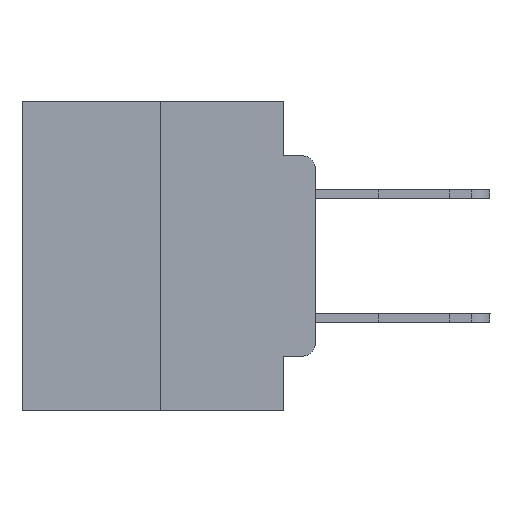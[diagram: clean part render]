
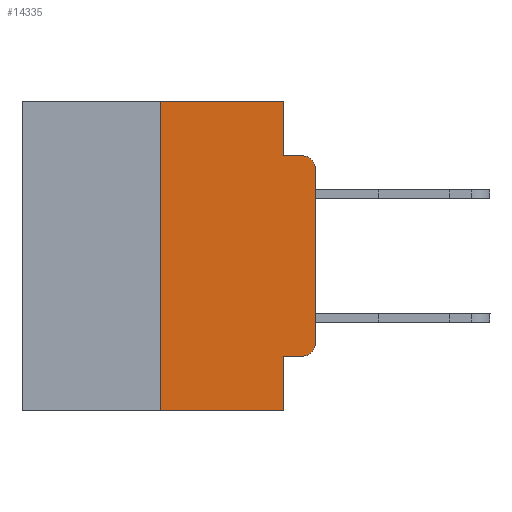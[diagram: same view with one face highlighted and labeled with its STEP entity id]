
A CAD part, left-side view. The second image highlights one B-rep face of the part: STEP entity #14335.
In plain terms, the highlighted planar face has unit normal (-1, 0, 0).
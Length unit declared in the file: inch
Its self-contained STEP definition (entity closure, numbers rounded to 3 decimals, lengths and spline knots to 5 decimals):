
#301 = CARTESIAN_POINT ( 'NONE',  ( 0., 0.051, -0.0885 ) ) ;
#1050 = CARTESIAN_POINT ( 'NONE',  ( 0., 0.02, -0.4115 ) ) ;
#1222 = DIRECTION ( 'NONE',  ( 0., -1., 0. ) ) ;
#1786 = VERTEX_POINT ( 'NONE', #24071 ) ;
#1843 = CARTESIAN_POINT ( 'NONE',  ( 0., 0.473, 0. ) ) ;
#1977 = ORIENTED_EDGE ( 'NONE', *, *, #16049, .F. ) ;
#2689 = LINE ( 'NONE', #21723, #15384 ) ;
#3329 = CARTESIAN_POINT ( 'NONE',  ( 0., 0.25, -0.5 ) ) ;
#3338 = DIRECTION ( 'NONE',  ( -1., 0., 0. ) ) ;
#4397 = VERTEX_POINT ( 'NONE', #22391 ) ;
#4562 = VERTEX_POINT ( 'NONE', #12631 ) ;
#4757 = VERTEX_POINT ( 'NONE', #17362 ) ;
#5115 = DIRECTION ( 'NONE',  ( 0., 0., -1. ) ) ;
#5194 = CARTESIAN_POINT ( 'NONE',  ( 0., 0.473, 0. ) ) ;
#5506 = EDGE_CURVE ( 'NONE', #17036, #4397, #13467, .T. ) ;
#5557 = CARTESIAN_POINT ( 'NONE',  ( 0., 0.25, 0. ) ) ;
#5837 = CARTESIAN_POINT ( 'NONE',  ( 0., 0.051, -0.4115 ) ) ;
#5929 = CARTESIAN_POINT ( 'NONE',  ( 0., 0.02, -0.1085 ) ) ;
#6880 = VECTOR ( 'NONE', #12243, 39.37008 ) ;
#7195 = CARTESIAN_POINT ( 'NONE',  ( 0., 0.25, 0. ) ) ;
#8250 = ORIENTED_EDGE ( 'NONE', *, *, #23955, .T. ) ;
#8496 = CARTESIAN_POINT ( 'NONE',  ( 0., 0.051, 0. ) ) ;
#9149 = AXIS2_PLACEMENT_3D ( 'NONE', #1843, #12012, #22225 ) ;
#9282 = VERTEX_POINT ( 'NONE', #17392 ) ;
#9330 = CARTESIAN_POINT ( 'NONE',  ( 0., 0.02, -0.0885 ) ) ;
#10525 = VECTOR ( 'NONE', #16918, 39.37008 ) ;
#11232 = ORIENTED_EDGE ( 'NONE', *, *, #19360, .T. ) ;
#11335 = VERTEX_POINT ( 'NONE', #7195 ) ;
#11630 = CARTESIAN_POINT ( 'NONE',  ( 0., 0.051, 0. ) ) ;
#11673 = DIRECTION ( 'NONE',  ( 0., 0., 1. ) ) ;
#11688 = VERTEX_POINT ( 'NONE', #9330 ) ;
#12012 = DIRECTION ( 'NONE',  ( 1., 0., 0. ) ) ;
#12243 = DIRECTION ( 'NONE',  ( 0., -1., 0. ) ) ;
#12631 = CARTESIAN_POINT ( 'NONE',  ( 0., 0.051, -0.4115 ) ) ;
#13405 = EDGE_CURVE ( 'NONE', #17850, #9282, #21242, .T. ) ;
#13409 = VECTOR ( 'NONE', #14598, 39.37008 ) ;
#13467 = CIRCLE ( 'NONE', #22019, 0.02 ) ;
#14068 = VECTOR ( 'NONE', #1222, 39.37008 ) ;
#14335 = ADVANCED_FACE ( 'NONE', ( #18044 ), #24498, .F. ) ;
#14598 = DIRECTION ( 'NONE',  ( 0., 0., -1. ) ) ;
#14749 = CARTESIAN_POINT ( 'NONE',  ( 0., 0., 0. ) ) ;
#14929 = EDGE_CURVE ( 'NONE', #9282, #11688, #19618, .T. ) ;
#15060 = VECTOR ( 'NONE', #20218, 39.37008 ) ;
#15384 = VECTOR ( 'NONE', #5115, 39.37008 ) ;
#15486 = VERTEX_POINT ( 'NONE', #3329 ) ;
#16049 = EDGE_CURVE ( 'NONE', #4562, #1786, #2689, .T. ) ;
#16918 = DIRECTION ( 'NONE',  ( 0., -1., 0. ) ) ;
#17036 = VERTEX_POINT ( 'NONE', #1050 ) ;
#17362 = CARTESIAN_POINT ( 'NONE',  ( 0., 0., -0.1085 ) ) ;
#17392 = CARTESIAN_POINT ( 'NONE',  ( 0., 0.051, -0.0885 ) ) ;
#17755 = CIRCLE ( 'NONE', #24842, 0.02 ) ;
#17850 = VERTEX_POINT ( 'NONE', #11630 ) ;
#17914 = EDGE_CURVE ( 'NONE', #4397, #4757, #22965, .T. ) ;
#17923 = DIRECTION ( 'NONE',  ( 0., 0., -1. ) ) ;
#18044 = FACE_OUTER_BOUND ( 'NONE', #19036, .T. ) ;
#18614 = VECTOR ( 'NONE', #11673, 39.37008 ) ;
#18925 = EDGE_CURVE ( 'NONE', #11335, #17850, #23853, .T. ) ;
#19036 = EDGE_LOOP ( 'NONE', ( #23358, #8250, #21638, #23681, #20014, #20599, #19217, #1977, #11232, #26768 ) ) ;
#19217 = ORIENTED_EDGE ( 'NONE', *, *, #21986, .T. ) ;
#19360 = EDGE_CURVE ( 'NONE', #4562, #17036, #22531, .T. ) ;
#19361 = VECTOR ( 'NONE', #22978, 39.37008 ) ;
#19618 = LINE ( 'NONE', #301, #10525 ) ;
#20014 = ORIENTED_EDGE ( 'NONE', *, *, #18925, .F. ) ;
#20218 = DIRECTION ( 'NONE',  ( 0., -1., 0. ) ) ;
#20487 = DIRECTION ( 'NONE',  ( -1., 0., 0. ) ) ;
#20599 = ORIENTED_EDGE ( 'NONE', *, *, #22430, .F. ) ;
#21242 = LINE ( 'NONE', #8496, #13409 ) ;
#21638 = ORIENTED_EDGE ( 'NONE', *, *, #14929, .F. ) ;
#21723 = CARTESIAN_POINT ( 'NONE',  ( 0., 0.051, 0. ) ) ;
#21986 = EDGE_CURVE ( 'NONE', #15486, #1786, #24850, .T. ) ;
#22019 = AXIS2_PLACEMENT_3D ( 'NONE', #26232, #3338, #17923 ) ;
#22225 = DIRECTION ( 'NONE',  ( 0., 0., -1. ) ) ;
#22344 = CARTESIAN_POINT ( 'NONE',  ( 0., 0.473, -0.5 ) ) ;
#22391 = CARTESIAN_POINT ( 'NONE',  ( 0., 0., -0.3915 ) ) ;
#22430 = EDGE_CURVE ( 'NONE', #15486, #11335, #24147, .T. ) ;
#22531 = LINE ( 'NONE', #5837, #6880 ) ;
#22965 = LINE ( 'NONE', #14749, #19361 ) ;
#22978 = DIRECTION ( 'NONE',  ( 0., 0., 1. ) ) ;
#23358 = ORIENTED_EDGE ( 'NONE', *, *, #17914, .T. ) ;
#23681 = ORIENTED_EDGE ( 'NONE', *, *, #13405, .F. ) ;
#23853 = LINE ( 'NONE', #5194, #14068 ) ;
#23955 = EDGE_CURVE ( 'NONE', #4757, #11688, #17755, .T. ) ;
#24071 = CARTESIAN_POINT ( 'NONE',  ( 0., 0.051, -0.5 ) ) ;
#24147 = LINE ( 'NONE', #5557, #18614 ) ;
#24498 = PLANE ( 'NONE',  #9149 ) ;
#24842 = AXIS2_PLACEMENT_3D ( 'NONE', #5929, #20487, #26351 ) ;
#24850 = LINE ( 'NONE', #22344, #15060 ) ;
#26232 = CARTESIAN_POINT ( 'NONE',  ( 0., 0.02, -0.3915 ) ) ;
#26351 = DIRECTION ( 'NONE',  ( 0., 0., -1. ) ) ;
#26768 = ORIENTED_EDGE ( 'NONE', *, *, #5506, .T. ) ;
